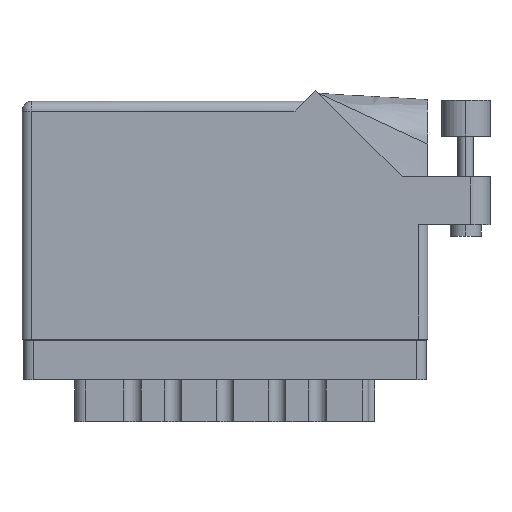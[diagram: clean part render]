
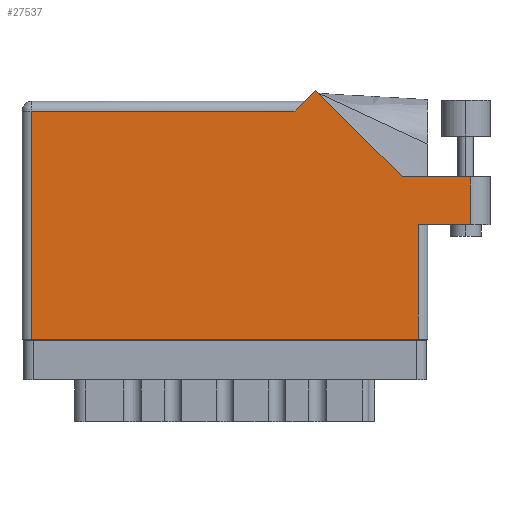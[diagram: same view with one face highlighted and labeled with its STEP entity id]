
A CAD part, front view. The second image highlights one B-rep face of the part: STEP entity #27537.
In plain terms, the highlighted face is planar.
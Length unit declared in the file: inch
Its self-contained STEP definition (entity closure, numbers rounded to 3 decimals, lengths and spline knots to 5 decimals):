
#36 = CARTESIAN_POINT ( 'NONE',  ( 1.88971, 1.60071, 0. ) ) ;
#41 = CARTESIAN_POINT ( 'NONE',  ( 2.887, 1.044, 0. ) ) ;
#214 = EDGE_CURVE ( 'NONE', #36428, #26362, #45338, .T. ) ;
#477 = CARTESIAN_POINT ( 'NONE',  ( 2.55, 0.737, 0. ) ) ;
#848 = ORIENTED_EDGE ( 'NONE', *, *, #27702, .T. ) ;
#2779 = DIRECTION ( 'NONE',  ( -1., 0., 0. ) ) ;
#3997 = ORIENTED_EDGE ( 'NONE', *, *, #10045, .T. ) ;
#4716 = VERTEX_POINT ( 'NONE', #33616 ) ;
#5672 = LINE ( 'NONE', #41191, #46983 ) ;
#7057 = VECTOR ( 'NONE', #10178, 39.37008 ) ;
#7176 = ORIENTED_EDGE ( 'NONE', *, *, #28763, .T. ) ;
#8025 = VECTOR ( 'NONE', #18928, 39.37008 ) ;
#8701 = ORIENTED_EDGE ( 'NONE', *, *, #23011, .T. ) ;
#10045 = EDGE_CURVE ( 'NONE', #22652, #12227, #37095, .T. ) ;
#10178 = DIRECTION ( 'NONE',  ( 1., 0., 0. ) ) ;
#11456 = VERTEX_POINT ( 'NONE', #15930 ) ;
#12227 = VERTEX_POINT ( 'NONE', #36 ) ;
#13349 = LINE ( 'NONE', #41, #8025 ) ;
#13802 = CARTESIAN_POINT ( 'NONE',  ( 3.012, 1.044, 0. ) ) ;
#14747 = LINE ( 'NONE', #33475, #34495 ) ;
#15155 = CARTESIAN_POINT ( 'NONE',  ( 2.44642, 1.044, 0. ) ) ;
#15326 = DIRECTION ( 'NONE',  ( -0.707, 0.707, 0. ) ) ;
#15770 = LINE ( 'NONE', #26543, #28374 ) ;
#15930 = CARTESIAN_POINT ( 'NONE',  ( 1.757, 1.468, 0. ) ) ;
#16022 = VECTOR ( 'NONE', #2779, 39.37008 ) ;
#17232 = VECTOR ( 'NONE', #19532, 39.37008 ) ;
#18928 = DIRECTION ( 'NONE',  ( 0., 1., 0. ) ) ;
#18946 = CARTESIAN_POINT ( 'NONE',  ( 2.55, 0.737, 0. ) ) ;
#19532 = DIRECTION ( 'NONE',  ( 0., 1., 0. ) ) ;
#20835 = LINE ( 'NONE', #13802, #16022 ) ;
#21590 = CARTESIAN_POINT ( 'NONE',  ( 0., 1.53, 0. ) ) ;
#21813 = CARTESIAN_POINT ( 'NONE',  ( 0.062, 1.468, 0. ) ) ;
#21818 = VECTOR ( 'NONE', #45205, 39.37008 ) ;
#22092 = ORIENTED_EDGE ( 'NONE', *, *, #31084, .T. ) ;
#22256 = PLANE ( 'NONE',  #27074 ) ;
#22652 = VERTEX_POINT ( 'NONE', #15155 ) ;
#23011 = EDGE_CURVE ( 'NONE', #11456, #43609, #5672, .T. ) ;
#23467 = VERTEX_POINT ( 'NONE', #18946 ) ;
#24972 = EDGE_CURVE ( 'NONE', #43609, #36428, #15770, .T. ) ;
#25178 = VECTOR ( 'NONE', #15326, 39.37008 ) ;
#25603 = CARTESIAN_POINT ( 'NONE',  ( 0., 0., 0. ) ) ;
#25762 = CARTESIAN_POINT ( 'NONE',  ( 2.55, 0., 0. ) ) ;
#25974 = DIRECTION ( 'NONE',  ( 1., 0., 0. ) ) ;
#26362 = VERTEX_POINT ( 'NONE', #25762 ) ;
#26543 = CARTESIAN_POINT ( 'NONE',  ( 0.062, 0., 0. ) ) ;
#27074 = AXIS2_PLACEMENT_3D ( 'NONE', #21590, #29747, #40935 ) ;
#27515 = FACE_OUTER_BOUND ( 'NONE', #33676, .T. ) ;
#27537 = ADVANCED_FACE ( 'NONE', ( #27515 ), #22256, .F. ) ;
#27702 = EDGE_CURVE ( 'NONE', #26362, #23467, #35204, .T. ) ;
#28374 = VECTOR ( 'NONE', #41572, 39.37008 ) ;
#28763 = EDGE_CURVE ( 'NONE', #42654, #22652, #20835, .T. ) ;
#29334 = EDGE_CURVE ( 'NONE', #23467, #4716, #14747, .T. ) ;
#29747 = DIRECTION ( 'NONE',  ( 0., 0., -1. ) ) ;
#30722 = CARTESIAN_POINT ( 'NONE',  ( 2.44642, 1.044, 0. ) ) ;
#31084 = EDGE_CURVE ( 'NONE', #4716, #42654, #13349, .T. ) ;
#31236 = ORIENTED_EDGE ( 'NONE', *, *, #214, .T. ) ;
#33475 = CARTESIAN_POINT ( 'NONE',  ( 2.612, 0.737, 0. ) ) ;
#33616 = CARTESIAN_POINT ( 'NONE',  ( 2.887, 0.737, 0. ) ) ;
#33676 = EDGE_LOOP ( 'NONE', ( #44061, #22092, #7176, #3997, #47846, #8701, #46395, #31236, #848 ) ) ;
#34495 = VECTOR ( 'NONE', #25974, 39.37008 ) ;
#35204 = LINE ( 'NONE', #477, #17232 ) ;
#36428 = VERTEX_POINT ( 'NONE', #41538 ) ;
#37095 = LINE ( 'NONE', #30722, #25178 ) ;
#40079 = CARTESIAN_POINT ( 'NONE',  ( 2.887, 1.044, 0. ) ) ;
#40935 = DIRECTION ( 'NONE',  ( -1., 0., 0. ) ) ;
#40960 = EDGE_CURVE ( 'NONE', #12227, #11456, #46351, .T. ) ;
#41191 = CARTESIAN_POINT ( 'NONE',  ( 0., 1.468, 0. ) ) ;
#41346 = CARTESIAN_POINT ( 'NONE',  ( 1.819, 1.53, 0. ) ) ;
#41538 = CARTESIAN_POINT ( 'NONE',  ( 0.062, 0., 0. ) ) ;
#41572 = DIRECTION ( 'NONE',  ( 0., -1., 0. ) ) ;
#42229 = DIRECTION ( 'NONE',  ( -1., 0., 0. ) ) ;
#42654 = VERTEX_POINT ( 'NONE', #40079 ) ;
#43609 = VERTEX_POINT ( 'NONE', #21813 ) ;
#44061 = ORIENTED_EDGE ( 'NONE', *, *, #29334, .T. ) ;
#45205 = DIRECTION ( 'NONE',  ( -0.707, -0.707, 0. ) ) ;
#45338 = LINE ( 'NONE', #25603, #7057 ) ;
#46351 = LINE ( 'NONE', #41346, #21818 ) ;
#46395 = ORIENTED_EDGE ( 'NONE', *, *, #24972, .T. ) ;
#46983 = VECTOR ( 'NONE', #42229, 39.37008 ) ;
#47846 = ORIENTED_EDGE ( 'NONE', *, *, #40960, .T. ) ;
